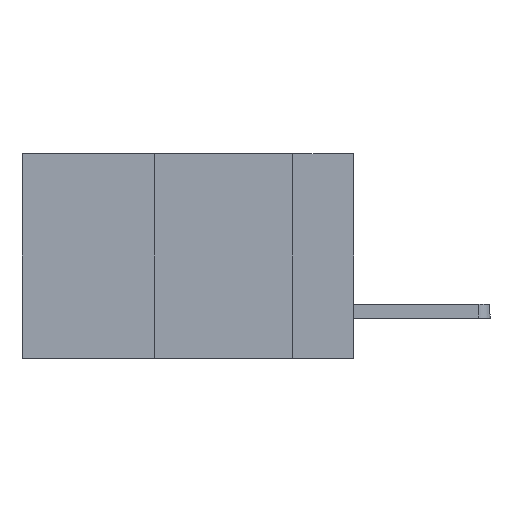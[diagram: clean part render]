
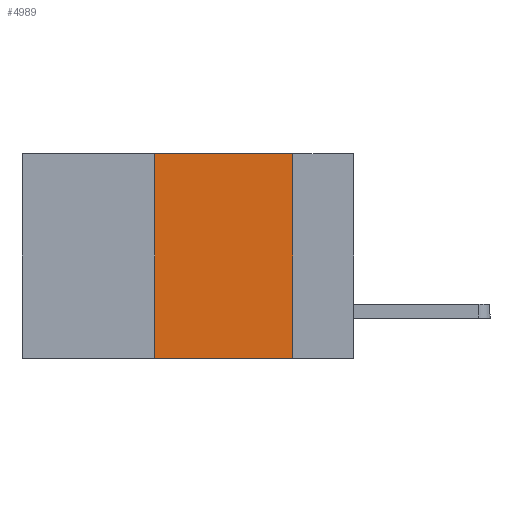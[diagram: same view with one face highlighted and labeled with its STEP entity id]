
A CAD part, left-side view. The second image highlights one B-rep face of the part: STEP entity #4989.
In plain terms, the highlighted planar face has unit normal (-1, 0, 0).
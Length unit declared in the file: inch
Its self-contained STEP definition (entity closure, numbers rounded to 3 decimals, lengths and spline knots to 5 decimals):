
#316 = EDGE_CURVE ( 'NONE', #2502, #5257, #4576, .T. ) ;
#457 = VERTEX_POINT ( 'NONE', #8192 ) ;
#1234 = CARTESIAN_POINT ( 'NONE',  ( 0., 0.11, 0. ) ) ;
#1290 = VECTOR ( 'NONE', #5517, 39.37008 ) ;
#1298 = AXIS2_PLACEMENT_3D ( 'NONE', #6170, #2728, #2717 ) ;
#1616 = CARTESIAN_POINT ( 'NONE',  ( 0., 0.36, -0.37 ) ) ;
#2461 = CARTESIAN_POINT ( 'NONE',  ( 0., 0.36, 0. ) ) ;
#2502 = VERTEX_POINT ( 'NONE', #1616 ) ;
#2717 = DIRECTION ( 'NONE',  ( 0., 0., -1. ) ) ;
#2728 = DIRECTION ( 'NONE',  ( 1., 0., 0. ) ) ;
#3643 = EDGE_CURVE ( 'NONE', #2502, #3758, #3803, .T. ) ;
#3758 = VERTEX_POINT ( 'NONE', #7107 ) ;
#3803 = LINE ( 'NONE', #9076, #7590 ) ;
#4049 = ORIENTED_EDGE ( 'NONE', *, *, #9436, .F. ) ;
#4321 = ORIENTED_EDGE ( 'NONE', *, *, #9128, .F. ) ;
#4576 = LINE ( 'NONE', #2461, #5818 ) ;
#4989 = ADVANCED_FACE ( 'NONE', ( #6899 ), #7246, .F. ) ;
#5081 = VECTOR ( 'NONE', #5748, 39.37008 ) ;
#5257 = VERTEX_POINT ( 'NONE', #6604 ) ;
#5517 = DIRECTION ( 'NONE',  ( 0., -1., 0. ) ) ;
#5748 = DIRECTION ( 'NONE',  ( 0., 0., -1. ) ) ;
#5818 = VECTOR ( 'NONE', #8167, 39.37008 ) ;
#6170 = CARTESIAN_POINT ( 'NONE',  ( 0., 0.6, 0. ) ) ;
#6515 = EDGE_LOOP ( 'NONE', ( #4321, #4049, #6859, #9000 ) ) ;
#6604 = CARTESIAN_POINT ( 'NONE',  ( 0., 0.36, 0. ) ) ;
#6859 = ORIENTED_EDGE ( 'NONE', *, *, #316, .F. ) ;
#6899 = FACE_OUTER_BOUND ( 'NONE', #6515, .T. ) ;
#6980 = DIRECTION ( 'NONE',  ( 0., -1., 0. ) ) ;
#6989 = LINE ( 'NONE', #1234, #5081 ) ;
#7107 = CARTESIAN_POINT ( 'NONE',  ( 0., 0.11, -0.37 ) ) ;
#7246 = PLANE ( 'NONE',  #1298 ) ;
#7590 = VECTOR ( 'NONE', #6980, 39.37008 ) ;
#7623 = CARTESIAN_POINT ( 'NONE',  ( 0., 0.6, 0. ) ) ;
#8167 = DIRECTION ( 'NONE',  ( 0., 0., 1. ) ) ;
#8192 = CARTESIAN_POINT ( 'NONE',  ( 0., 0.11, 0. ) ) ;
#8923 = LINE ( 'NONE', #7623, #1290 ) ;
#9000 = ORIENTED_EDGE ( 'NONE', *, *, #3643, .T. ) ;
#9076 = CARTESIAN_POINT ( 'NONE',  ( 0., 0.6, -0.37 ) ) ;
#9128 = EDGE_CURVE ( 'NONE', #457, #3758, #6989, .T. ) ;
#9436 = EDGE_CURVE ( 'NONE', #5257, #457, #8923, .T. ) ;
